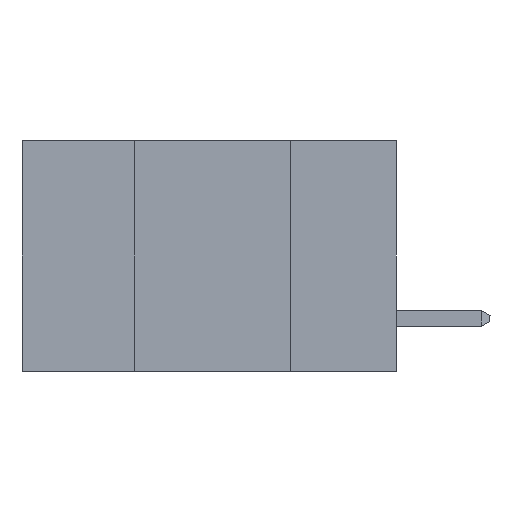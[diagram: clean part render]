
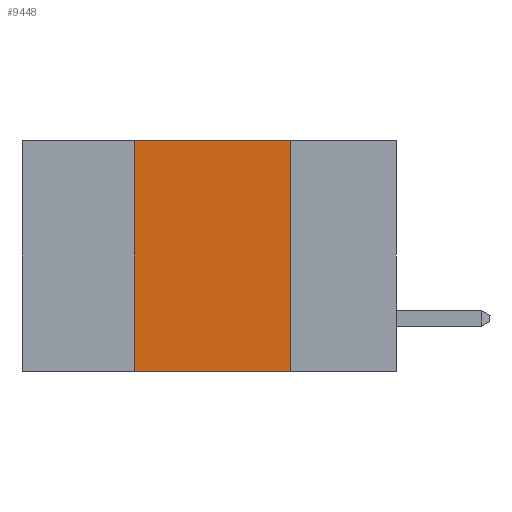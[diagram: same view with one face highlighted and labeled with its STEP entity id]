
A CAD part, left-side view. The second image highlights one B-rep face of the part: STEP entity #9448.
In plain terms, the highlighted planar face has unit normal (-1, 0, 0).
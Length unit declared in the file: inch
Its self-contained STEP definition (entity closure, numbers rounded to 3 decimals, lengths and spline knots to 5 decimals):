
#1078 = CARTESIAN_POINT ( 'NONE',  ( 0., 0.17, -0.37 ) ) ;
#1531 = ORIENTED_EDGE ( 'NONE', *, *, #4655, .F. ) ;
#1546 = LINE ( 'NONE', #1078, #10321 ) ;
#1604 = VERTEX_POINT ( 'NONE', #6927 ) ;
#1933 = EDGE_CURVE ( 'NONE', #9847, #1604, #1546, .T. ) ;
#2076 = PLANE ( 'NONE',  #3510 ) ;
#3080 = DIRECTION ( 'NONE',  ( 1., 0., 0. ) ) ;
#3510 = AXIS2_PLACEMENT_3D ( 'NONE', #8303, #3080, #9091 ) ;
#4035 = VERTEX_POINT ( 'NONE', #8213 ) ;
#4303 = ORIENTED_EDGE ( 'NONE', *, *, #1933, .F. ) ;
#4492 = EDGE_CURVE ( 'NONE', #4035, #1604, #11328, .T. ) ;
#4637 = DIRECTION ( 'NONE',  ( 0., 0., -1. ) ) ;
#4655 = EDGE_CURVE ( 'NONE', #11150, #9847, #6761, .T. ) ;
#4666 = DIRECTION ( 'NONE',  ( 0., 0., 1. ) ) ;
#4747 = CARTESIAN_POINT ( 'NONE',  ( 0., 0.42, -0.37 ) ) ;
#5595 = FACE_OUTER_BOUND ( 'NONE', #6234, .T. ) ;
#6234 = EDGE_LOOP ( 'NONE', ( #4303, #1531, #6328, #6767 ) ) ;
#6328 = ORIENTED_EDGE ( 'NONE', *, *, #7000, .F. ) ;
#6545 = CARTESIAN_POINT ( 'NONE',  ( 0., 0.6, 0. ) ) ;
#6698 = DIRECTION ( 'NONE',  ( 0., -1., 0. ) ) ;
#6761 = LINE ( 'NONE', #6545, #10945 ) ;
#6767 = ORIENTED_EDGE ( 'NONE', *, *, #4492, .T. ) ;
#6927 = CARTESIAN_POINT ( 'NONE',  ( 0., 0.17, -0.37 ) ) ;
#7000 = EDGE_CURVE ( 'NONE', #4035, #11150, #8211, .T. ) ;
#8211 = LINE ( 'NONE', #4747, #10396 ) ;
#8213 = CARTESIAN_POINT ( 'NONE',  ( 0., 0.42, -0.37 ) ) ;
#8303 = CARTESIAN_POINT ( 'NONE',  ( 0., 0.6, 0. ) ) ;
#8354 = DIRECTION ( 'NONE',  ( 0., -1., 0. ) ) ;
#8587 = CARTESIAN_POINT ( 'NONE',  ( 0., 0.6, -0.37 ) ) ;
#8753 = CARTESIAN_POINT ( 'NONE',  ( 0., 0.42, 0. ) ) ;
#9091 = DIRECTION ( 'NONE',  ( 0., 0., -1. ) ) ;
#9448 = ADVANCED_FACE ( 'NONE', ( #5595 ), #2076, .F. ) ;
#9847 = VERTEX_POINT ( 'NONE', #10509 ) ;
#10321 = VECTOR ( 'NONE', #4637, 39.37008 ) ;
#10396 = VECTOR ( 'NONE', #4666, 39.37008 ) ;
#10509 = CARTESIAN_POINT ( 'NONE',  ( 0., 0.17, 0. ) ) ;
#10815 = VECTOR ( 'NONE', #8354, 39.37008 ) ;
#10945 = VECTOR ( 'NONE', #6698, 39.37008 ) ;
#11150 = VERTEX_POINT ( 'NONE', #8753 ) ;
#11328 = LINE ( 'NONE', #8587, #10815 ) ;
